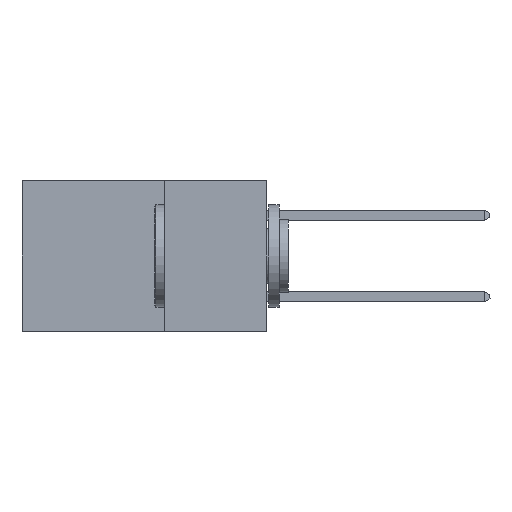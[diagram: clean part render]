
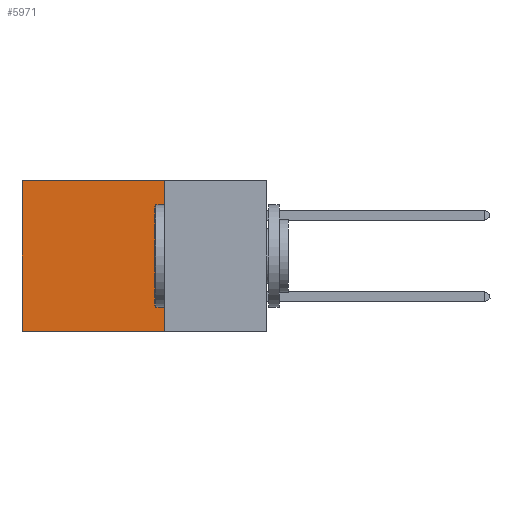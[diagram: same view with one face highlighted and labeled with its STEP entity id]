
A CAD part, left-side view. The second image highlights one B-rep face of the part: STEP entity #5971.
In plain terms, the highlighted planar face has unit normal (-1, 0, 0).
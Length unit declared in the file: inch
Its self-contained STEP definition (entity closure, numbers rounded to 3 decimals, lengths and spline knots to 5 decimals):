
#543 = LINE ( 'NONE', #9483, #1062 ) ;
#1062 = VECTOR ( 'NONE', #17739, 39.37008 ) ;
#1941 = VERTEX_POINT ( 'NONE', #6870 ) ;
#2154 = DIRECTION ( 'NONE',  ( 0., 1., 0. ) ) ;
#2178 = ORIENTED_EDGE ( 'NONE', *, *, #8922, .T. ) ;
#2938 = VERTEX_POINT ( 'NONE', #4261 ) ;
#3099 = CARTESIAN_POINT ( 'NONE',  ( 0.2875, 0.25, -0.37 ) ) ;
#3112 = VERTEX_POINT ( 'NONE', #17529 ) ;
#4261 = CARTESIAN_POINT ( 'NONE',  ( 0.2875, 0.6, -0.37 ) ) ;
#4674 = LINE ( 'NONE', #15284, #15672 ) ;
#5971 = ADVANCED_FACE ( 'NONE', ( #6433 ), #16881, .F. ) ;
#6433 = FACE_OUTER_BOUND ( 'NONE', #14820, .T. ) ;
#6597 = CARTESIAN_POINT ( 'NONE',  ( 0.2875, 0.25, 0. ) ) ;
#6870 = CARTESIAN_POINT ( 'NONE',  ( 0.2875, 0.25, -0.37 ) ) ;
#8922 = EDGE_CURVE ( 'NONE', #3112, #16455, #13089, .T. ) ;
#9483 = CARTESIAN_POINT ( 'NONE',  ( 0.2875, 0.25, 0. ) ) ;
#9678 = ORIENTED_EDGE ( 'NONE', *, *, #15805, .F. ) ;
#9972 = VECTOR ( 'NONE', #18662, 39.37008 ) ;
#10082 = DIRECTION ( 'NONE',  ( 0., 0., -1. ) ) ;
#10776 = AXIS2_PLACEMENT_3D ( 'NONE', #12829, #18266, #10082 ) ;
#11218 = DIRECTION ( 'NONE',  ( 0., 0., -1. ) ) ;
#11896 = EDGE_CURVE ( 'NONE', #1941, #2938, #18118, .T. ) ;
#12829 = CARTESIAN_POINT ( 'NONE',  ( 0.2875, 0.25, 0. ) ) ;
#12950 = ORIENTED_EDGE ( 'NONE', *, *, #14339, .T. ) ;
#13089 = LINE ( 'NONE', #6597, #16264 ) ;
#14339 = EDGE_CURVE ( 'NONE', #16455, #2938, #4674, .T. ) ;
#14762 = CARTESIAN_POINT ( 'NONE',  ( 0.2875, 0.6, 0. ) ) ;
#14820 = EDGE_LOOP ( 'NONE', ( #12950, #16550, #9678, #2178 ) ) ;
#15284 = CARTESIAN_POINT ( 'NONE',  ( 0.2875, 0.6, 0. ) ) ;
#15672 = VECTOR ( 'NONE', #11218, 39.37008 ) ;
#15805 = EDGE_CURVE ( 'NONE', #3112, #1941, #543, .T. ) ;
#16264 = VECTOR ( 'NONE', #2154, 39.37008 ) ;
#16455 = VERTEX_POINT ( 'NONE', #14762 ) ;
#16550 = ORIENTED_EDGE ( 'NONE', *, *, #11896, .F. ) ;
#16881 = PLANE ( 'NONE',  #10776 ) ;
#17529 = CARTESIAN_POINT ( 'NONE',  ( 0.2875, 0.25, 0. ) ) ;
#17739 = DIRECTION ( 'NONE',  ( 0., 0., -1. ) ) ;
#18118 = LINE ( 'NONE', #3099, #9972 ) ;
#18266 = DIRECTION ( 'NONE',  ( 1., 0., 0. ) ) ;
#18662 = DIRECTION ( 'NONE',  ( 0., 1., 0. ) ) ;
